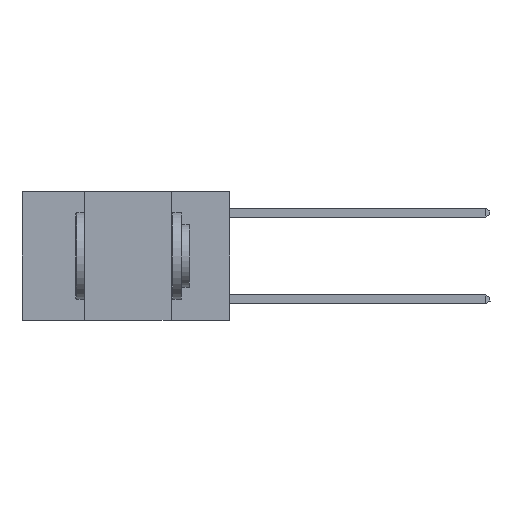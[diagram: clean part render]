
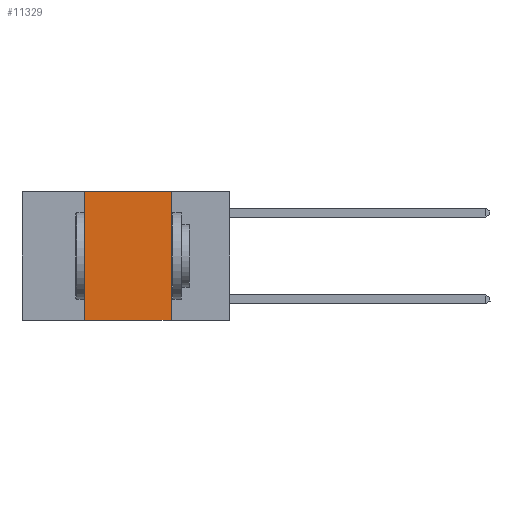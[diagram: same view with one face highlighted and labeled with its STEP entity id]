
A CAD part, left-side view. The second image highlights one B-rep face of the part: STEP entity #11329.
In plain terms, the highlighted planar face has unit normal (-1, 0, 0).
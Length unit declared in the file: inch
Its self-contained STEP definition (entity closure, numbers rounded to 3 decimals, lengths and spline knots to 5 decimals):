
#855 = AXIS2_PLACEMENT_3D ( 'NONE', #23366, #25430, #12855 ) ;
#2349 = VERTEX_POINT ( 'NONE', #16631 ) ;
#3526 = CARTESIAN_POINT ( 'NONE',  ( 0., 0.42, 0. ) ) ;
#4059 = VECTOR ( 'NONE', #13153, 39.37008 ) ;
#4146 = VECTOR ( 'NONE', #7981, 39.37008 ) ;
#4463 = CARTESIAN_POINT ( 'NONE',  ( 0., 0.17, 0. ) ) ;
#6258 = DIRECTION ( 'NONE',  ( 0., -1., 0. ) ) ;
#6838 = CARTESIAN_POINT ( 'NONE',  ( 0., 0.6, -0.37 ) ) ;
#7981 = DIRECTION ( 'NONE',  ( 0., 0., 1. ) ) ;
#9040 = DIRECTION ( 'NONE',  ( 0., -1., 0. ) ) ;
#9043 = LINE ( 'NONE', #17038, #14095 ) ;
#9332 = VERTEX_POINT ( 'NONE', #11564 ) ;
#10055 = VERTEX_POINT ( 'NONE', #13713 ) ;
#11165 = ORIENTED_EDGE ( 'NONE', *, *, #13342, .F. ) ;
#11284 = VERTEX_POINT ( 'NONE', #14826 ) ;
#11329 = ADVANCED_FACE ( 'NONE', ( #17928 ), #21273, .F. ) ;
#11347 = ORIENTED_EDGE ( 'NONE', *, *, #27526, .F. ) ;
#11564 = CARTESIAN_POINT ( 'NONE',  ( 0., 0.17, -0.37 ) ) ;
#11865 = EDGE_CURVE ( 'NONE', #10055, #11284, #27651, .T. ) ;
#12855 = DIRECTION ( 'NONE',  ( 0., 0., -1. ) ) ;
#13153 = DIRECTION ( 'NONE',  ( 0., 0., -1. ) ) ;
#13342 = EDGE_CURVE ( 'NONE', #2349, #9332, #16300, .T. ) ;
#13713 = CARTESIAN_POINT ( 'NONE',  ( 0., 0.42, -0.37 ) ) ;
#14095 = VECTOR ( 'NONE', #6258, 39.37008 ) ;
#14826 = CARTESIAN_POINT ( 'NONE',  ( 0., 0.42, 0. ) ) ;
#14937 = ORIENTED_EDGE ( 'NONE', *, *, #19028, .T. ) ;
#15060 = LINE ( 'NONE', #6838, #25527 ) ;
#16300 = LINE ( 'NONE', #4463, #4059 ) ;
#16631 = CARTESIAN_POINT ( 'NONE',  ( 0., 0.17, 0. ) ) ;
#17038 = CARTESIAN_POINT ( 'NONE',  ( 0., 0.6, 0. ) ) ;
#17871 = ORIENTED_EDGE ( 'NONE', *, *, #11865, .F. ) ;
#17928 = FACE_OUTER_BOUND ( 'NONE', #24505, .T. ) ;
#19028 = EDGE_CURVE ( 'NONE', #10055, #9332, #15060, .T. ) ;
#21273 = PLANE ( 'NONE',  #855 ) ;
#23366 = CARTESIAN_POINT ( 'NONE',  ( 0., 0.6, 0. ) ) ;
#24505 = EDGE_LOOP ( 'NONE', ( #11165, #11347, #17871, #14937 ) ) ;
#25430 = DIRECTION ( 'NONE',  ( 1., 0., 0. ) ) ;
#25527 = VECTOR ( 'NONE', #9040, 39.37008 ) ;
#27526 = EDGE_CURVE ( 'NONE', #11284, #2349, #9043, .T. ) ;
#27651 = LINE ( 'NONE', #3526, #4146 ) ;
